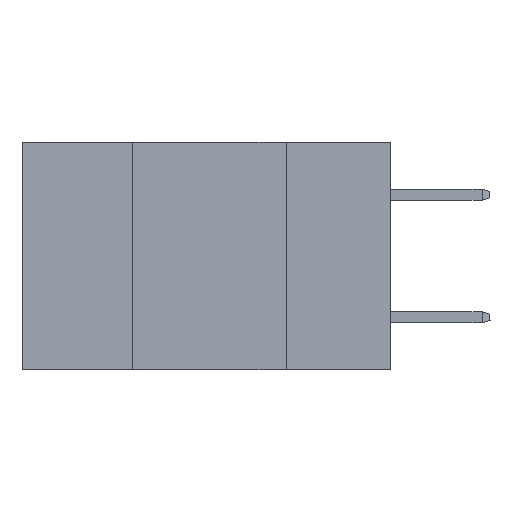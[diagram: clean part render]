
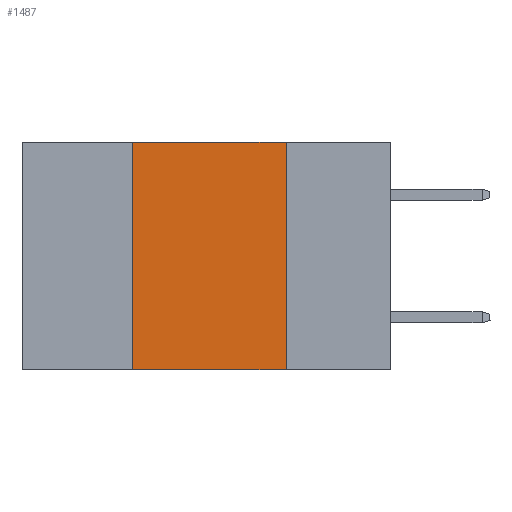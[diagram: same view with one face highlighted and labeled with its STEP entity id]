
A CAD part, left-side view. The second image highlights one B-rep face of the part: STEP entity #1487.
In plain terms, the highlighted planar face has unit normal (-1, 0, 0).
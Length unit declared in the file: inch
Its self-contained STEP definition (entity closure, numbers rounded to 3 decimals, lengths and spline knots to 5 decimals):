
#45 = DIRECTION ( 'NONE',  ( 0., 0., -1. ) ) ;
#93 = CARTESIAN_POINT ( 'NONE',  ( 0., 0.42, 0. ) ) ;
#401 = DIRECTION ( 'NONE',  ( 0., 0., 1. ) ) ;
#431 = LINE ( 'NONE', #4591, #9481 ) ;
#1487 = ADVANCED_FACE ( 'NONE', ( #6443 ), #8339, .F. ) ;
#1577 = ORIENTED_EDGE ( 'NONE', *, *, #4200, .F. ) ;
#1751 = AXIS2_PLACEMENT_3D ( 'NONE', #6298, #10614, #45 ) ;
#1776 = LINE ( 'NONE', #9009, #8760 ) ;
#2179 = EDGE_CURVE ( 'NONE', #3150, #3556, #2866, .T. ) ;
#2375 = LINE ( 'NONE', #7671, #6454 ) ;
#2866 = LINE ( 'NONE', #8040, #3058 ) ;
#2974 = EDGE_CURVE ( 'NONE', #3556, #3445, #1776, .T. ) ;
#3058 = VECTOR ( 'NONE', #10023, 39.37008 ) ;
#3150 = VERTEX_POINT ( 'NONE', #93 ) ;
#3445 = VERTEX_POINT ( 'NONE', #12087 ) ;
#3556 = VERTEX_POINT ( 'NONE', #12545 ) ;
#3642 = ORIENTED_EDGE ( 'NONE', *, *, #11843, .T. ) ;
#3767 = ORIENTED_EDGE ( 'NONE', *, *, #2179, .F. ) ;
#4200 = EDGE_CURVE ( 'NONE', #6812, #3150, #2375, .T. ) ;
#4591 = CARTESIAN_POINT ( 'NONE',  ( 0., 0.6, -0.37 ) ) ;
#6298 = CARTESIAN_POINT ( 'NONE',  ( 0., 0.6, 0. ) ) ;
#6443 = FACE_OUTER_BOUND ( 'NONE', #8536, .T. ) ;
#6454 = VECTOR ( 'NONE', #401, 39.37008 ) ;
#6812 = VERTEX_POINT ( 'NONE', #8571 ) ;
#7169 = DIRECTION ( 'NONE',  ( 0., 0., -1. ) ) ;
#7671 = CARTESIAN_POINT ( 'NONE',  ( 0., 0.42, 0. ) ) ;
#7778 = DIRECTION ( 'NONE',  ( 0., -1., 0. ) ) ;
#8040 = CARTESIAN_POINT ( 'NONE',  ( 0., 0.6, 0. ) ) ;
#8339 = PLANE ( 'NONE',  #1751 ) ;
#8536 = EDGE_LOOP ( 'NONE', ( #12671, #3767, #1577, #3642 ) ) ;
#8571 = CARTESIAN_POINT ( 'NONE',  ( 0., 0.42, -0.37 ) ) ;
#8760 = VECTOR ( 'NONE', #7169, 39.37008 ) ;
#9009 = CARTESIAN_POINT ( 'NONE',  ( 0., 0.17, 0. ) ) ;
#9481 = VECTOR ( 'NONE', #7778, 39.37008 ) ;
#10023 = DIRECTION ( 'NONE',  ( 0., -1., 0. ) ) ;
#10614 = DIRECTION ( 'NONE',  ( 1., 0., 0. ) ) ;
#11843 = EDGE_CURVE ( 'NONE', #6812, #3445, #431, .T. ) ;
#12087 = CARTESIAN_POINT ( 'NONE',  ( 0., 0.17, -0.37 ) ) ;
#12545 = CARTESIAN_POINT ( 'NONE',  ( 0., 0.17, 0. ) ) ;
#12671 = ORIENTED_EDGE ( 'NONE', *, *, #2974, .F. ) ;
